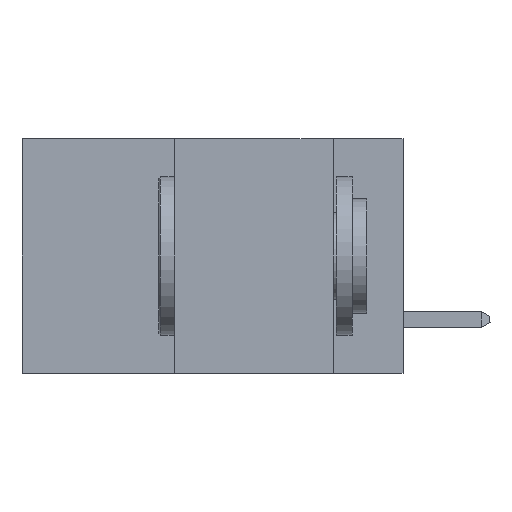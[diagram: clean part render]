
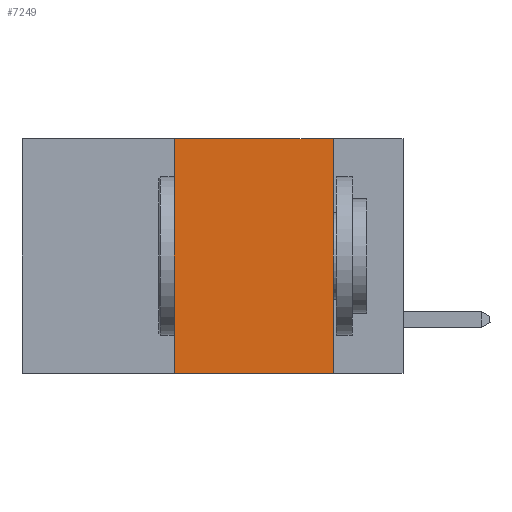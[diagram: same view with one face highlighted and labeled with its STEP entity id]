
A CAD part, left-side view. The second image highlights one B-rep face of the part: STEP entity #7249.
In plain terms, the highlighted planar face has unit normal (-1, 0, 0).
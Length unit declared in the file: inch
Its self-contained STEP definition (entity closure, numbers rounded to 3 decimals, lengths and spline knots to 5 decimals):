
#55 = LINE ( 'NONE', #26534, #38420 ) ;
#396 = DIRECTION ( 'NONE',  ( 0., 0., -1. ) ) ;
#428 = VECTOR ( 'NONE', #18626, 39.37008 ) ;
#741 = EDGE_CURVE ( 'NONE', #13609, #27023, #7465, .T. ) ;
#1805 = DIRECTION ( 'NONE',  ( 0., -1., 0. ) ) ;
#2704 = CARTESIAN_POINT ( 'NONE',  ( 0., 0.11, -0.37 ) ) ;
#5339 = DIRECTION ( 'NONE',  ( 0., -1., 0. ) ) ;
#5511 = ORIENTED_EDGE ( 'NONE', *, *, #28444, .F. ) ;
#7222 = LINE ( 'NONE', #38046, #30507 ) ;
#7249 = ADVANCED_FACE ( 'NONE', ( #12387 ), #15585, .F. ) ;
#7465 = LINE ( 'NONE', #17380, #15554 ) ;
#9473 = CARTESIAN_POINT ( 'NONE',  ( 0., 0.6, 0. ) ) ;
#12387 = FACE_OUTER_BOUND ( 'NONE', #33381, .T. ) ;
#13609 = VERTEX_POINT ( 'NONE', #33609 ) ;
#15554 = VECTOR ( 'NONE', #16732, 39.37008 ) ;
#15558 = CARTESIAN_POINT ( 'NONE',  ( 0., 0.11, 0. ) ) ;
#15585 = PLANE ( 'NONE',  #26941 ) ;
#16732 = DIRECTION ( 'NONE',  ( 0., 0., 1. ) ) ;
#16778 = ORIENTED_EDGE ( 'NONE', *, *, #33550, .F. ) ;
#17380 = CARTESIAN_POINT ( 'NONE',  ( 0., 0.36, 0. ) ) ;
#18626 = DIRECTION ( 'NONE',  ( 0., 0., -1. ) ) ;
#18650 = DIRECTION ( 'NONE',  ( 1., 0., 0. ) ) ;
#18772 = ORIENTED_EDGE ( 'NONE', *, *, #27377, .T. ) ;
#25558 = VERTEX_POINT ( 'NONE', #2704 ) ;
#26284 = ORIENTED_EDGE ( 'NONE', *, *, #741, .F. ) ;
#26534 = CARTESIAN_POINT ( 'NONE',  ( 0., 0.6, 0. ) ) ;
#26941 = AXIS2_PLACEMENT_3D ( 'NONE', #9473, #18650, #396 ) ;
#27023 = VERTEX_POINT ( 'NONE', #27957 ) ;
#27377 = EDGE_CURVE ( 'NONE', #13609, #25558, #7222, .T. ) ;
#27957 = CARTESIAN_POINT ( 'NONE',  ( 0., 0.36, 0. ) ) ;
#28444 = EDGE_CURVE ( 'NONE', #34647, #25558, #31817, .T. ) ;
#29156 = CARTESIAN_POINT ( 'NONE',  ( 0., 0.11, 0. ) ) ;
#30507 = VECTOR ( 'NONE', #1805, 39.37008 ) ;
#31817 = LINE ( 'NONE', #15558, #428 ) ;
#33381 = EDGE_LOOP ( 'NONE', ( #5511, #16778, #26284, #18772 ) ) ;
#33550 = EDGE_CURVE ( 'NONE', #27023, #34647, #55, .T. ) ;
#33609 = CARTESIAN_POINT ( 'NONE',  ( 0., 0.36, -0.37 ) ) ;
#34647 = VERTEX_POINT ( 'NONE', #29156 ) ;
#38046 = CARTESIAN_POINT ( 'NONE',  ( 0., 0.6, -0.37 ) ) ;
#38420 = VECTOR ( 'NONE', #5339, 39.37008 ) ;
